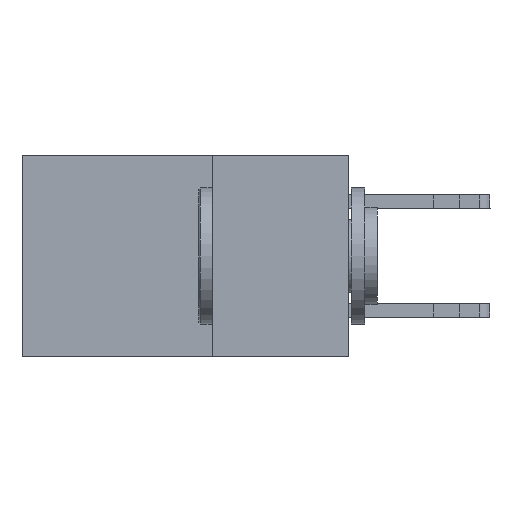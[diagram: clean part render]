
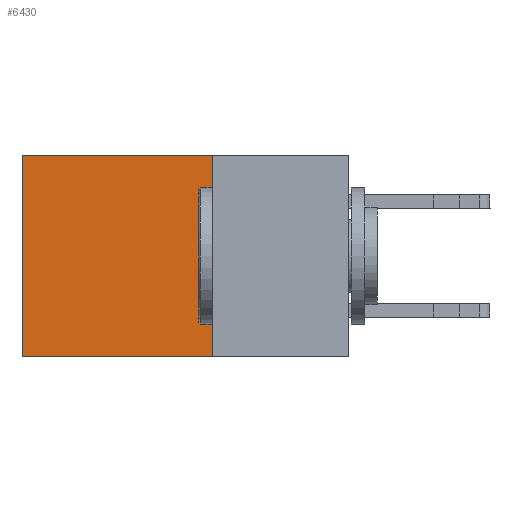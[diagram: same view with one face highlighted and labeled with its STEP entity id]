
A CAD part, left-side view. The second image highlights one B-rep face of the part: STEP entity #6430.
In plain terms, the highlighted planar face has unit normal (-1, 0, 0).
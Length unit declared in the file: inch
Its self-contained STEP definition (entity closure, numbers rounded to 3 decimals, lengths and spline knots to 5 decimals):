
#36 = ORIENTED_EDGE ( 'NONE', *, *, #6556, .T. ) ;
#78 = VERTEX_POINT ( 'NONE', #3357 ) ;
#312 = EDGE_LOOP ( 'NONE', ( #9177, #5861, #11638, #36 ) ) ;
#608 = VECTOR ( 'NONE', #11307, 39.37008 ) ;
#751 = DIRECTION ( 'NONE',  ( 1., 0., 0. ) ) ;
#1317 = CARTESIAN_POINT ( 'NONE',  ( 0.2615, 0.25, -0.37 ) ) ;
#2179 = DIRECTION ( 'NONE',  ( 0., 1., 0. ) ) ;
#2312 = LINE ( 'NONE', #1317, #10677 ) ;
#2855 = LINE ( 'NONE', #11248, #608 ) ;
#3179 = VERTEX_POINT ( 'NONE', #5451 ) ;
#3357 = CARTESIAN_POINT ( 'NONE',  ( 0.2615, 0.6, 0. ) ) ;
#3536 = FACE_OUTER_BOUND ( 'NONE', #312, .T. ) ;
#3578 = CARTESIAN_POINT ( 'NONE',  ( 0.2615, 0.25, -0.37 ) ) ;
#3782 = EDGE_CURVE ( 'NONE', #78, #7900, #6594, .T. ) ;
#3886 = DIRECTION ( 'NONE',  ( 0., 0., -1. ) ) ;
#4327 = DIRECTION ( 'NONE',  ( 0., 0., -1. ) ) ;
#5368 = LINE ( 'NONE', #3578, #11662 ) ;
#5451 = CARTESIAN_POINT ( 'NONE',  ( 0.2615, 0.25, -0.37 ) ) ;
#5552 = AXIS2_PLACEMENT_3D ( 'NONE', #6553, #751, #9335 ) ;
#5861 = ORIENTED_EDGE ( 'NONE', *, *, #6852, .F. ) ;
#6430 = ADVANCED_FACE ( 'NONE', ( #3536 ), #11134, .F. ) ;
#6553 = CARTESIAN_POINT ( 'NONE',  ( 0.2615, 0.25, -0.37 ) ) ;
#6556 = EDGE_CURVE ( 'NONE', #7321, #78, #2855, .T. ) ;
#6594 = LINE ( 'NONE', #6657, #8046 ) ;
#6657 = CARTESIAN_POINT ( 'NONE',  ( 0.2615, 0.6, -0.37 ) ) ;
#6852 = EDGE_CURVE ( 'NONE', #3179, #7900, #2312, .T. ) ;
#7321 = VERTEX_POINT ( 'NONE', #9133 ) ;
#7345 = EDGE_CURVE ( 'NONE', #7321, #3179, #5368, .T. ) ;
#7900 = VERTEX_POINT ( 'NONE', #8552 ) ;
#8046 = VECTOR ( 'NONE', #3886, 39.37008 ) ;
#8552 = CARTESIAN_POINT ( 'NONE',  ( 0.2615, 0.6, -0.37 ) ) ;
#9133 = CARTESIAN_POINT ( 'NONE',  ( 0.2615, 0.25, 0. ) ) ;
#9177 = ORIENTED_EDGE ( 'NONE', *, *, #3782, .T. ) ;
#9335 = DIRECTION ( 'NONE',  ( 0., 0., -1. ) ) ;
#10677 = VECTOR ( 'NONE', #2179, 39.37008 ) ;
#11134 = PLANE ( 'NONE',  #5552 ) ;
#11248 = CARTESIAN_POINT ( 'NONE',  ( 0.2615, 0.25, 0. ) ) ;
#11307 = DIRECTION ( 'NONE',  ( 0., 1., 0. ) ) ;
#11638 = ORIENTED_EDGE ( 'NONE', *, *, #7345, .F. ) ;
#11662 = VECTOR ( 'NONE', #4327, 39.37008 ) ;
